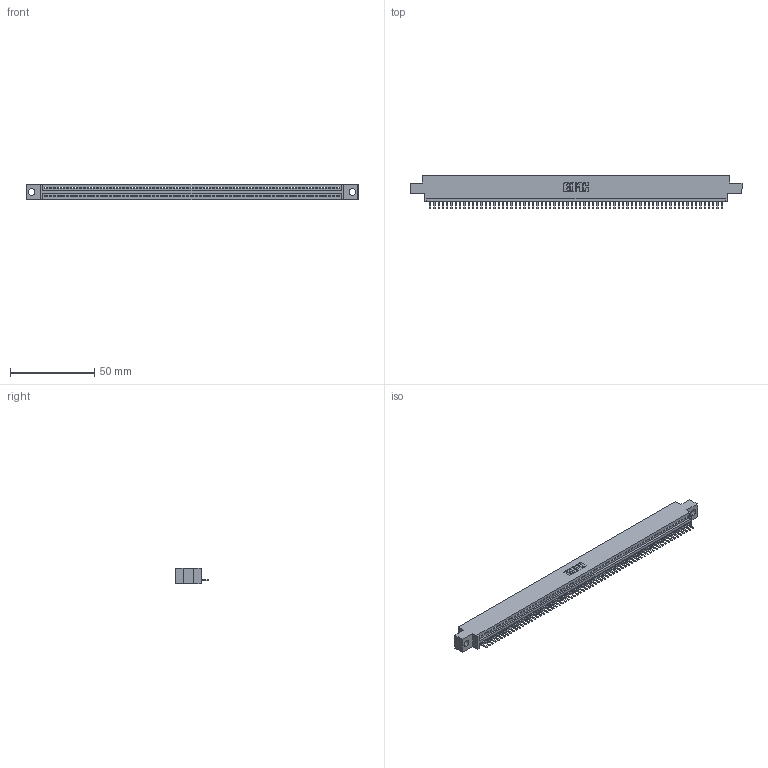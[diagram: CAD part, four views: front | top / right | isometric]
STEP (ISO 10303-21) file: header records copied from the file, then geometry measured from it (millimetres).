
FILE_DESCRIPTION (( 'STEP AP203' ), '1' );
FILE_NAME ('345-069-520-604.STEP', '2021-05-28T16:17:34', ( '' ), ( '' ), 'SwSTEP 2.0', 'SolidWorks 2020', '' );
FILE_SCHEMA (( 'CONFIG_CONTROL_DESIGN' ));
Length unit declared in the file: inch
Products named in the file (3): 345-069-520-604; 345 Part_0.170 Offset - 0.156 Dia-TI; 345-292-001_345-293-120
Assembly tree (70 placements, depth 2):
  345-069-520-604
    345 Part_0.170 Offset - 0.156 Dia-TI
    345-292-001_345-293-120  x69
Bounding box: 196.47 x 19.68 x 9.4 mm (x, y, z)
Volume: 18464.2 mm3; surface area: 24223.9 mm2
Topology: 70 solids, 70 shells, 4422 faces, 13085 edges, 8538 vertices
Faces by surface type: plane 2996, cylinder 1426
Entity records: 48961 total; most frequent: CARTESIAN_POINT 8501, ORIENTED_EDGE 8490, DIRECTION 7371, EDGE_CURVE 4245, LINE 3833, VECTOR 3833, VERTEX_POINT 2826, AXIS2_PLACEMENT_3D 1769
